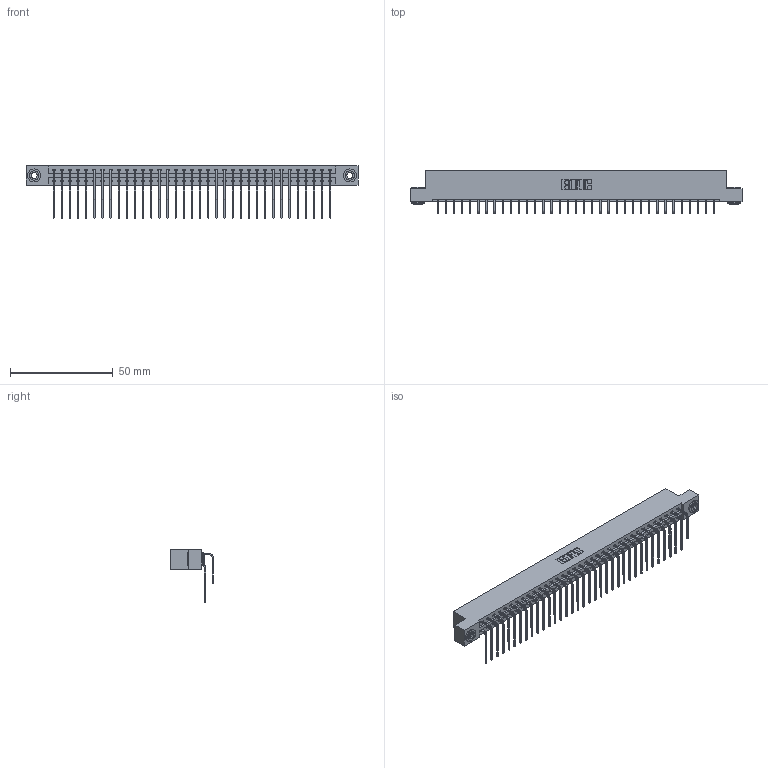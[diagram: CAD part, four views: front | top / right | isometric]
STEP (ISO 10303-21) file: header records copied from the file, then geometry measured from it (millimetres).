
FILE_DESCRIPTION (( 'STEP AP203' ), '1' );
FILE_NAME ('337-070-559-203.STEP', '2018-08-11T13:19:46', ( '' ), ( '' ), 'SwSTEP 2.0', 'SolidWorks 2016', '' );
FILE_SCHEMA (( 'CONFIG_CONTROL_DESIGN' ));
Length unit declared in the file: inch
Products named in the file (5): 337 Part_Flush Mounting Lugs - 0.156 Dia-TH; 345-292-001_558 559 Tail - 1; 345-292-001_559 Tail - 2; 345-250-002_345-250-002-102; 337-070-559-203
Assembly tree (73 placements, depth 2):
  337-070-559-203
    337 Part_Flush Mounting Lugs - 0.156 Dia-TH
    345-292-001_558 559 Tail - 1  x35
    345-292-001_559 Tail - 2  x35
    345-250-002_345-250-002-102  x2
Bounding box: 161.7 x 20.9 x 25.53 mm (x, y, z)
Volume: 17370.9 mm3; surface area: 21821.8 mm2
Topology: 73 solids, 73 shells, 4072 faces, 12077 edges, 7954 vertices
Faces by surface type: plane 2880, cylinder 1184, cone 8
Entity records: 30476 total; most frequent: CARTESIAN_POINT 5160, ORIENTED_EDGE 5038, DIRECTION 4417, EDGE_CURVE 2519, LINE 2327, VECTOR 2327, VERTEX_POINT 1674, AXIS2_PLACEMENT_3D 1045
